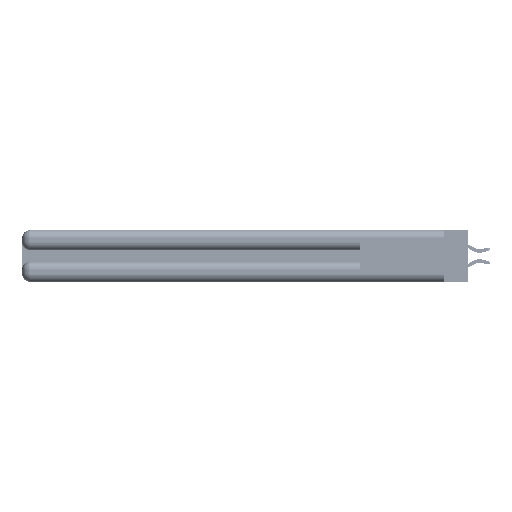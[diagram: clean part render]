
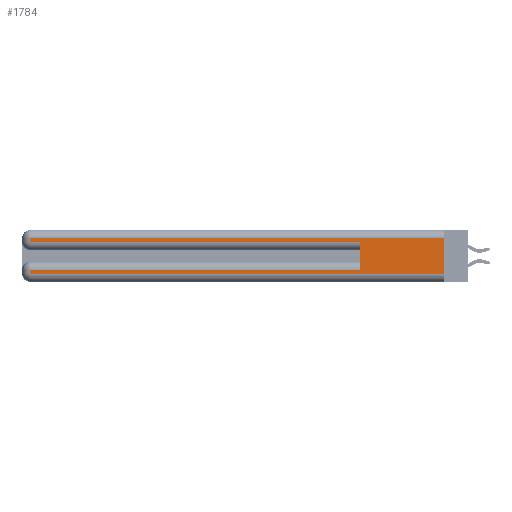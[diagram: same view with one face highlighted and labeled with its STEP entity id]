
A CAD part, left-side view. The second image highlights one B-rep face of the part: STEP entity #1784.
In plain terms, the highlighted planar face has unit normal (-1, 0, 0).
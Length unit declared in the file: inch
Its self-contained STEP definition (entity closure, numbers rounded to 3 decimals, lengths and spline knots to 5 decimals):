
#810 = DIRECTION ( 'NONE',  ( 0., 0., 1. ) ) ;
#1784 = ADVANCED_FACE ( 'NONE', ( #38003 ), #7435, .F. ) ;
#1833 = CARTESIAN_POINT ( 'NONE',  ( 0., 0., 0.31 ) ) ;
#2037 = VECTOR ( 'NONE', #45348, 39.37008 ) ;
#3914 = VECTOR ( 'NONE', #5824, 39.37008 ) ;
#5824 = DIRECTION ( 'NONE',  ( 0., 0., -1. ) ) ;
#6189 = CARTESIAN_POINT ( 'NONE',  ( 0., 0., 0.37 ) ) ;
#6928 = DIRECTION ( 'NONE',  ( 0., 0., -1. ) ) ;
#7435 = PLANE ( 'NONE',  #48925 ) ;
#8774 = LINE ( 'NONE', #6189, #12446 ) ;
#9860 = VECTOR ( 'NONE', #39636, 39.37008 ) ;
#10370 = ORIENTED_EDGE ( 'NONE', *, *, #39494, .F. ) ;
#12446 = VECTOR ( 'NONE', #48830, 39.37008 ) ;
#13485 = VECTOR ( 'NONE', #49279, 39.37008 ) ;
#13961 = ORIENTED_EDGE ( 'NONE', *, *, #32490, .F. ) ;
#15277 = CARTESIAN_POINT ( 'NONE',  ( 0., 0., 0.06 ) ) ;
#15663 = VERTEX_POINT ( 'NONE', #45702 ) ;
#16376 = LINE ( 'NONE', #29961, #2037 ) ;
#16958 = LINE ( 'NONE', #49107, #39728 ) ;
#17560 = CARTESIAN_POINT ( 'NONE',  ( 0., 0.6, 0.085 ) ) ;
#18540 = VERTEX_POINT ( 'NONE', #28332 ) ;
#18636 = DIRECTION ( 'NONE',  ( 1., 0., 0. ) ) ;
#19678 = VERTEX_POINT ( 'NONE', #34221 ) ;
#19681 = VECTOR ( 'NONE', #30085, 39.37008 ) ;
#22408 = ORIENTED_EDGE ( 'NONE', *, *, #43642, .T. ) ;
#23696 = EDGE_CURVE ( 'NONE', #31084, #28041, #16376, .T. ) ;
#26066 = VECTOR ( 'NONE', #810, 39.37008 ) ;
#26136 = DIRECTION ( 'NONE',  ( 0., 0., -1. ) ) ;
#26630 = EDGE_CURVE ( 'NONE', #33750, #36761, #40034, .T. ) ;
#26963 = EDGE_CURVE ( 'NONE', #15663, #28635, #43383, .T. ) ;
#27739 = CARTESIAN_POINT ( 'NONE',  ( 0., 2.94, 0.285 ) ) ;
#28041 = VERTEX_POINT ( 'NONE', #48897 ) ;
#28332 = CARTESIAN_POINT ( 'NONE',  ( 0., 0., 0.06 ) ) ;
#28635 = VERTEX_POINT ( 'NONE', #38990 ) ;
#28709 = CARTESIAN_POINT ( 'NONE',  ( 0., 2.94, 0.37 ) ) ;
#28931 = EDGE_LOOP ( 'NONE', ( #10370, #37358, #22408, #39355, #13961, #39047, #47257, #48699 ) ) ;
#29001 = LINE ( 'NONE', #15277, #13485 ) ;
#29961 = CARTESIAN_POINT ( 'NONE',  ( 0., 0., 0.285 ) ) ;
#30085 = DIRECTION ( 'NONE',  ( 0., 1., 0. ) ) ;
#30375 = CARTESIAN_POINT ( 'NONE',  ( 0., 2.94, 0.085 ) ) ;
#30742 = CARTESIAN_POINT ( 'NONE',  ( 0., 0., 0.085 ) ) ;
#30877 = CARTESIAN_POINT ( 'NONE',  ( 0., 0.6, 0.145 ) ) ;
#31084 = VERTEX_POINT ( 'NONE', #27739 ) ;
#32490 = EDGE_CURVE ( 'NONE', #33750, #28041, #42271, .T. ) ;
#33750 = VERTEX_POINT ( 'NONE', #17560 ) ;
#34221 = CARTESIAN_POINT ( 'NONE',  ( 0., 2.94, 0.06 ) ) ;
#34489 = EDGE_CURVE ( 'NONE', #36761, #19678, #38046, .T. ) ;
#34714 = EDGE_CURVE ( 'NONE', #19678, #18540, #29001, .T. ) ;
#36761 = VERTEX_POINT ( 'NONE', #30375 ) ;
#37358 = ORIENTED_EDGE ( 'NONE', *, *, #26963, .T. ) ;
#38003 = FACE_OUTER_BOUND ( 'NONE', #28931, .T. ) ;
#38046 = LINE ( 'NONE', #28709, #3914 ) ;
#38990 = CARTESIAN_POINT ( 'NONE',  ( 0., 2.94, 0.31 ) ) ;
#39047 = ORIENTED_EDGE ( 'NONE', *, *, #26630, .T. ) ;
#39355 = ORIENTED_EDGE ( 'NONE', *, *, #23696, .T. ) ;
#39494 = EDGE_CURVE ( 'NONE', #15663, #18540, #8774, .T. ) ;
#39636 = DIRECTION ( 'NONE',  ( 0., 1., 0. ) ) ;
#39728 = VECTOR ( 'NONE', #26136, 39.37008 ) ;
#40034 = LINE ( 'NONE', #30742, #19681 ) ;
#41380 = CARTESIAN_POINT ( 'NONE',  ( 0., 0., 0.37 ) ) ;
#42271 = LINE ( 'NONE', #30877, #26066 ) ;
#43383 = LINE ( 'NONE', #1833, #9860 ) ;
#43642 = EDGE_CURVE ( 'NONE', #28635, #31084, #16958, .T. ) ;
#45348 = DIRECTION ( 'NONE',  ( 0., -1., 0. ) ) ;
#45702 = CARTESIAN_POINT ( 'NONE',  ( 0., 0., 0.31 ) ) ;
#47257 = ORIENTED_EDGE ( 'NONE', *, *, #34489, .T. ) ;
#48699 = ORIENTED_EDGE ( 'NONE', *, *, #34714, .T. ) ;
#48830 = DIRECTION ( 'NONE',  ( 0., 0., -1. ) ) ;
#48897 = CARTESIAN_POINT ( 'NONE',  ( 0., 0.6, 0.285 ) ) ;
#48925 = AXIS2_PLACEMENT_3D ( 'NONE', #41380, #18636, #6928 ) ;
#49107 = CARTESIAN_POINT ( 'NONE',  ( 0., 2.94, 0.37 ) ) ;
#49279 = DIRECTION ( 'NONE',  ( 0., -1., 0. ) ) ;
